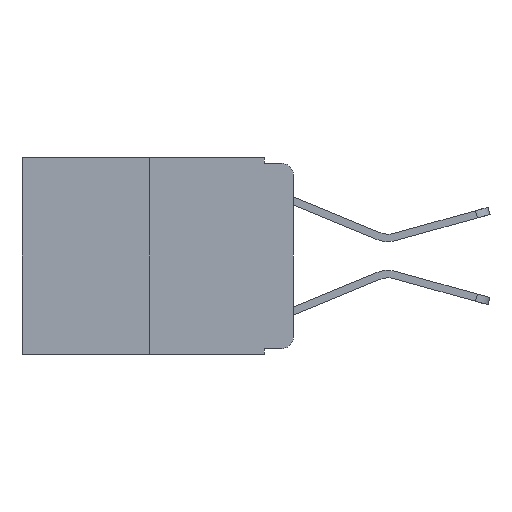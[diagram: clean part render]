
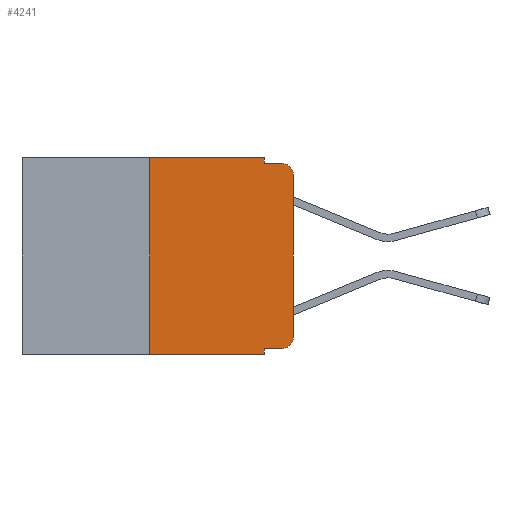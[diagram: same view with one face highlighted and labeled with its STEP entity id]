
A CAD part, left-side view. The second image highlights one B-rep face of the part: STEP entity #4241.
In plain terms, the highlighted planar face has unit normal (-1, 0, 0).
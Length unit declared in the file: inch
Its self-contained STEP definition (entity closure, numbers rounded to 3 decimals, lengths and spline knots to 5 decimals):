
#341 = CARTESIAN_POINT ( 'NONE',  ( 0., 0., 0. ) ) ;
#832 = CARTESIAN_POINT ( 'NONE',  ( 0., 0.051, 0. ) ) ;
#1393 = DIRECTION ( 'NONE',  ( 0., -1., 0. ) ) ;
#1467 = DIRECTION ( 'NONE',  ( 0., 0., 1. ) ) ;
#1802 = ORIENTED_EDGE ( 'NONE', *, *, #11999, .F. ) ;
#2147 = EDGE_CURVE ( 'NONE', #3737, #11195, #6260, .T. ) ;
#2256 = ORIENTED_EDGE ( 'NONE', *, *, #12658, .T. ) ;
#2333 = VECTOR ( 'NONE', #20180, 39.37008 ) ;
#3023 = DIRECTION ( 'NONE',  ( 0., 0., -1. ) ) ;
#3042 = DIRECTION ( 'NONE',  ( 0., -1., 0. ) ) ;
#3540 = EDGE_LOOP ( 'NONE', ( #16073, #2256, #4878, #5213, #18551, #18226, #12727, #1802, #6471, #18984 ) ) ;
#3541 = DIRECTION ( 'NONE',  ( 0., 0., -1. ) ) ;
#3695 = EDGE_CURVE ( 'NONE', #6158, #3737, #4616, .T. ) ;
#3737 = VERTEX_POINT ( 'NONE', #832 ) ;
#3798 = AXIS2_PLACEMENT_3D ( 'NONE', #9260, #20532, #10934 ) ;
#3968 = CARTESIAN_POINT ( 'NONE',  ( 0., 0.051, -0.01 ) ) ;
#4101 = VECTOR ( 'NONE', #3042, 39.37008 ) ;
#4241 = ADVANCED_FACE ( 'NONE', ( #6966 ), #20945, .F. ) ;
#4616 = LINE ( 'NONE', #21271, #4101 ) ;
#4802 = VECTOR ( 'NONE', #10599, 39.37008 ) ;
#4878 = ORIENTED_EDGE ( 'NONE', *, *, #5264, .F. ) ;
#4908 = CARTESIAN_POINT ( 'NONE',  ( 0., 0.051, -0.333 ) ) ;
#4937 = VERTEX_POINT ( 'NONE', #11462 ) ;
#4998 = CIRCLE ( 'NONE', #3798, 0.02 ) ;
#5138 = CARTESIAN_POINT ( 'NONE',  ( 0., 0.02, -0.01 ) ) ;
#5213 = ORIENTED_EDGE ( 'NONE', *, *, #2147, .F. ) ;
#5264 = EDGE_CURVE ( 'NONE', #11195, #19740, #5330, .T. ) ;
#5287 = LINE ( 'NONE', #6961, #13545 ) ;
#5330 = LINE ( 'NONE', #3968, #4802 ) ;
#5505 = CARTESIAN_POINT ( 'NONE',  ( 0., 0., -0.313 ) ) ;
#6158 = VERTEX_POINT ( 'NONE', #14641 ) ;
#6205 = AXIS2_PLACEMENT_3D ( 'NONE', #16563, #6818, #18188 ) ;
#6260 = LINE ( 'NONE', #11304, #9643 ) ;
#6471 = ORIENTED_EDGE ( 'NONE', *, *, #12535, .T. ) ;
#6610 = DIRECTION ( 'NONE',  ( 0., -1., 0. ) ) ;
#6685 = VECTOR ( 'NONE', #1393, 39.37008 ) ;
#6818 = DIRECTION ( 'NONE',  ( -1., 0., 0. ) ) ;
#6840 = LINE ( 'NONE', #341, #2333 ) ;
#6958 = DIRECTION ( 'NONE',  ( 0., 0., -1. ) ) ;
#6961 = CARTESIAN_POINT ( 'NONE',  ( 0., 0.051, 0. ) ) ;
#6966 = FACE_OUTER_BOUND ( 'NONE', #3540, .T. ) ;
#7370 = VECTOR ( 'NONE', #1467, 39.37008 ) ;
#7619 = LINE ( 'NONE', #4908, #15780 ) ;
#7705 = EDGE_CURVE ( 'NONE', #8886, #14350, #6840, .T. ) ;
#7920 = CARTESIAN_POINT ( 'NONE',  ( 0., 0.25, -0.343 ) ) ;
#8562 = VERTEX_POINT ( 'NONE', #7920 ) ;
#8886 = VERTEX_POINT ( 'NONE', #5505 ) ;
#9260 = CARTESIAN_POINT ( 'NONE',  ( 0., 0.02, -0.03 ) ) ;
#9539 = CIRCLE ( 'NONE', #6205, 0.02 ) ;
#9643 = VECTOR ( 'NONE', #6958, 39.37008 ) ;
#9682 = CARTESIAN_POINT ( 'NONE',  ( 0., 0.02, -0.333 ) ) ;
#9983 = VERTEX_POINT ( 'NONE', #9682 ) ;
#10599 = DIRECTION ( 'NONE',  ( 0., -1., 0. ) ) ;
#10721 = CARTESIAN_POINT ( 'NONE',  ( 0., 0.051, -0.333 ) ) ;
#10934 = DIRECTION ( 'NONE',  ( 0., 0., -1. ) ) ;
#11195 = VERTEX_POINT ( 'NONE', #16211 ) ;
#11304 = CARTESIAN_POINT ( 'NONE',  ( 0., 0.051, 0. ) ) ;
#11356 = CARTESIAN_POINT ( 'NONE',  ( 0., 0.473, 0. ) ) ;
#11462 = CARTESIAN_POINT ( 'NONE',  ( 0., 0.051, -0.343 ) ) ;
#11999 = EDGE_CURVE ( 'NONE', #20649, #4937, #5287, .T. ) ;
#12263 = LINE ( 'NONE', #17918, #7370 ) ;
#12535 = EDGE_CURVE ( 'NONE', #20649, #9983, #7619, .T. ) ;
#12658 = EDGE_CURVE ( 'NONE', #14350, #19740, #4998, .T. ) ;
#12727 = ORIENTED_EDGE ( 'NONE', *, *, #19638, .T. ) ;
#12827 = AXIS2_PLACEMENT_3D ( 'NONE', #11356, #12975, #3023 ) ;
#12975 = DIRECTION ( 'NONE',  ( 1., 0., 0. ) ) ;
#13545 = VECTOR ( 'NONE', #3541, 39.37008 ) ;
#14179 = EDGE_CURVE ( 'NONE', #9983, #8886, #9539, .T. ) ;
#14347 = LINE ( 'NONE', #21055, #6685 ) ;
#14350 = VERTEX_POINT ( 'NONE', #15430 ) ;
#14641 = CARTESIAN_POINT ( 'NONE',  ( 0., 0.25, 0. ) ) ;
#15430 = CARTESIAN_POINT ( 'NONE',  ( 0., 0., -0.03 ) ) ;
#15780 = VECTOR ( 'NONE', #6610, 39.37008 ) ;
#16064 = EDGE_CURVE ( 'NONE', #8562, #6158, #12263, .T. ) ;
#16073 = ORIENTED_EDGE ( 'NONE', *, *, #7705, .T. ) ;
#16211 = CARTESIAN_POINT ( 'NONE',  ( 0., 0.051, -0.01 ) ) ;
#16563 = CARTESIAN_POINT ( 'NONE',  ( 0., 0.02, -0.313 ) ) ;
#17918 = CARTESIAN_POINT ( 'NONE',  ( 0., 0.25, 0. ) ) ;
#18188 = DIRECTION ( 'NONE',  ( 0., 0., -1. ) ) ;
#18226 = ORIENTED_EDGE ( 'NONE', *, *, #16064, .F. ) ;
#18551 = ORIENTED_EDGE ( 'NONE', *, *, #3695, .F. ) ;
#18984 = ORIENTED_EDGE ( 'NONE', *, *, #14179, .T. ) ;
#19638 = EDGE_CURVE ( 'NONE', #8562, #4937, #14347, .T. ) ;
#19740 = VERTEX_POINT ( 'NONE', #5138 ) ;
#20180 = DIRECTION ( 'NONE',  ( 0., 0., 1. ) ) ;
#20532 = DIRECTION ( 'NONE',  ( -1., 0., 0. ) ) ;
#20649 = VERTEX_POINT ( 'NONE', #10721 ) ;
#20945 = PLANE ( 'NONE',  #12827 ) ;
#21055 = CARTESIAN_POINT ( 'NONE',  ( 0., 0.473, -0.343 ) ) ;
#21271 = CARTESIAN_POINT ( 'NONE',  ( 0., 0.473, 0. ) ) ;
